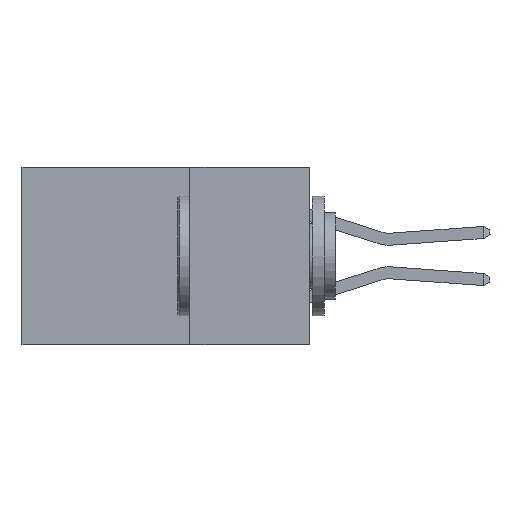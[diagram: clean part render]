
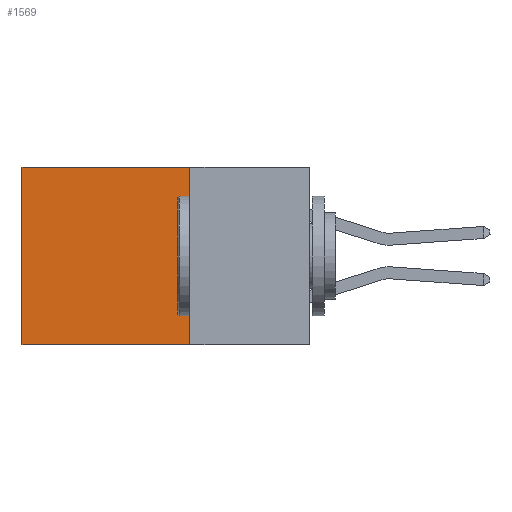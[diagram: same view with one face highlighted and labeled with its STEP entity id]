
A CAD part, left-side view. The second image highlights one B-rep face of the part: STEP entity #1569.
In plain terms, the highlighted planar face has unit normal (-1, 0, 0).
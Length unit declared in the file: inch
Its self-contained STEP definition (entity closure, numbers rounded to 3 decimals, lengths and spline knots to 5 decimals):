
#126 = LINE ( 'NONE', #2887, #6824 ) ;
#208 = CARTESIAN_POINT ( 'NONE',  ( 0.2615, 0.25, -0.37 ) ) ;
#235 = CARTESIAN_POINT ( 'NONE',  ( 0.2615, 0.25, -0.37 ) ) ;
#865 = VECTOR ( 'NONE', #8325, 39.37008 ) ;
#1569 = ADVANCED_FACE ( 'NONE', ( #5592 ), #11106, .F. ) ;
#2341 = DIRECTION ( 'NONE',  ( 0., 1., 0. ) ) ;
#2712 = CARTESIAN_POINT ( 'NONE',  ( 0.2615, 0.25, -0.37 ) ) ;
#2803 = ORIENTED_EDGE ( 'NONE', *, *, #5082, .F. ) ;
#2887 = CARTESIAN_POINT ( 'NONE',  ( 0.2615, 0.6, -0.37 ) ) ;
#3413 = VECTOR ( 'NONE', #10274, 39.37008 ) ;
#3921 = AXIS2_PLACEMENT_3D ( 'NONE', #2712, #4754, #5544 ) ;
#4106 = EDGE_CURVE ( 'NONE', #4666, #5576, #6772, .T. ) ;
#4279 = LINE ( 'NONE', #10569, #5183 ) ;
#4379 = ORIENTED_EDGE ( 'NONE', *, *, #7316, .T. ) ;
#4651 = CARTESIAN_POINT ( 'NONE',  ( 0.2615, 0.25, 0. ) ) ;
#4666 = VERTEX_POINT ( 'NONE', #4651 ) ;
#4754 = DIRECTION ( 'NONE',  ( 1., 0., 0. ) ) ;
#4810 = LINE ( 'NONE', #235, #3413 ) ;
#5017 = CARTESIAN_POINT ( 'NONE',  ( 0.2615, 0.6, -0.37 ) ) ;
#5082 = EDGE_CURVE ( 'NONE', #5576, #5637, #4810, .T. ) ;
#5183 = VECTOR ( 'NONE', #2341, 39.37008 ) ;
#5490 = DIRECTION ( 'NONE',  ( 0., 0., -1. ) ) ;
#5492 = ORIENTED_EDGE ( 'NONE', *, *, #6561, .T. ) ;
#5544 = DIRECTION ( 'NONE',  ( 0., 0., -1. ) ) ;
#5576 = VERTEX_POINT ( 'NONE', #208 ) ;
#5592 = FACE_OUTER_BOUND ( 'NONE', #7978, .T. ) ;
#5637 = VERTEX_POINT ( 'NONE', #5017 ) ;
#6400 = ORIENTED_EDGE ( 'NONE', *, *, #4106, .F. ) ;
#6561 = EDGE_CURVE ( 'NONE', #4666, #11185, #4279, .T. ) ;
#6772 = LINE ( 'NONE', #9287, #865 ) ;
#6824 = VECTOR ( 'NONE', #5490, 39.37008 ) ;
#7316 = EDGE_CURVE ( 'NONE', #11185, #5637, #126, .T. ) ;
#7874 = CARTESIAN_POINT ( 'NONE',  ( 0.2615, 0.6, 0. ) ) ;
#7978 = EDGE_LOOP ( 'NONE', ( #4379, #2803, #6400, #5492 ) ) ;
#8325 = DIRECTION ( 'NONE',  ( 0., 0., -1. ) ) ;
#9287 = CARTESIAN_POINT ( 'NONE',  ( 0.2615, 0.25, -0.37 ) ) ;
#10274 = DIRECTION ( 'NONE',  ( 0., 1., 0. ) ) ;
#10569 = CARTESIAN_POINT ( 'NONE',  ( 0.2615, 0.25, 0. ) ) ;
#11106 = PLANE ( 'NONE',  #3921 ) ;
#11185 = VERTEX_POINT ( 'NONE', #7874 ) ;
